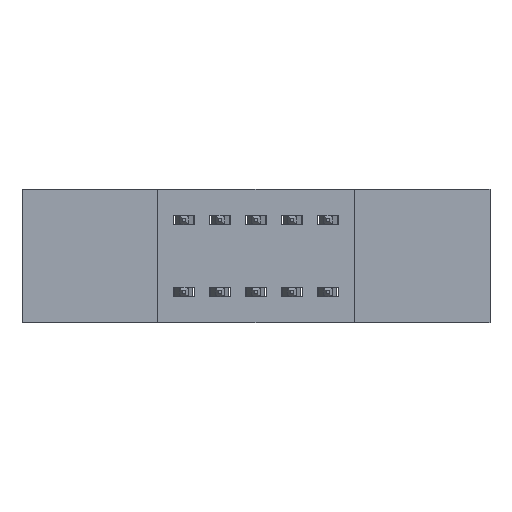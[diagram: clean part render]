
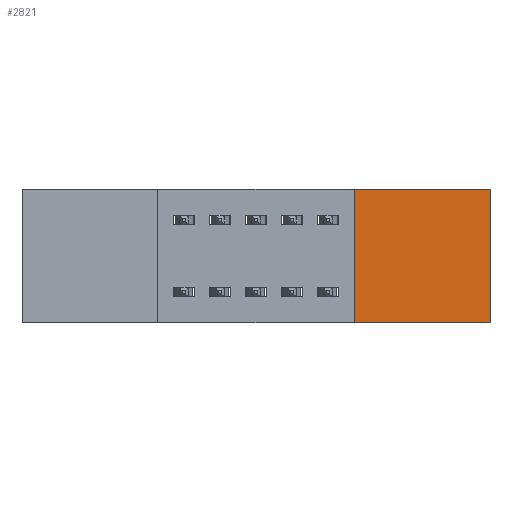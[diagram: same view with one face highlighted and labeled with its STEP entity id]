
A CAD part, front view. The second image highlights one B-rep face of the part: STEP entity #2821.
In plain terms, the highlighted planar face has unit normal (0, -1, 0).
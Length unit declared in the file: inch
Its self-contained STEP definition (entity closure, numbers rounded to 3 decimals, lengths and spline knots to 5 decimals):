
#245 = ORIENTED_EDGE ( 'NONE', *, *, #5132, .F. ) ;
#257 = VECTOR ( 'NONE', #2340, 39.37008 ) ;
#269 = FACE_OUTER_BOUND ( 'NONE', #7204, .T. ) ;
#697 = ORIENTED_EDGE ( 'NONE', *, *, #5958, .F. ) ;
#896 = EDGE_CURVE ( 'NONE', #3418, #1655, #3836, .T. ) ;
#955 = PLANE ( 'NONE',  #3244 ) ;
#995 = CARTESIAN_POINT ( 'NONE',  ( 0., 0., -0.37 ) ) ;
#1147 = VERTEX_POINT ( 'NONE', #1577 ) ;
#1577 = CARTESIAN_POINT ( 'NONE',  ( 0.923, 0., 0. ) ) ;
#1655 = VERTEX_POINT ( 'NONE', #2865 ) ;
#1747 = LINE ( 'NONE', #2254, #7863 ) ;
#2162 = DIRECTION ( 'NONE',  ( 0., -1., 0. ) ) ;
#2254 = CARTESIAN_POINT ( 'NONE',  ( 0., 0., 0. ) ) ;
#2340 = DIRECTION ( 'NONE',  ( 0., 0., -1. ) ) ;
#2496 = CARTESIAN_POINT ( 'NONE',  ( 0., 0., -0.37 ) ) ;
#2521 = ORIENTED_EDGE ( 'NONE', *, *, #4552, .F. ) ;
#2821 = ADVANCED_FACE ( 'NONE', ( #269 ), #955, .T. ) ;
#2865 = CARTESIAN_POINT ( 'NONE',  ( 1.3, 0., -0.37 ) ) ;
#3244 = AXIS2_PLACEMENT_3D ( 'NONE', #2496, #2162, #5313 ) ;
#3418 = VERTEX_POINT ( 'NONE', #5886 ) ;
#3768 = CARTESIAN_POINT ( 'NONE',  ( 0.923, 0., -0.37 ) ) ;
#3836 = LINE ( 'NONE', #4072, #257 ) ;
#4072 = CARTESIAN_POINT ( 'NONE',  ( 1.3, 0., 0. ) ) ;
#4094 = VECTOR ( 'NONE', #7202, 39.37008 ) ;
#4458 = DIRECTION ( 'NONE',  ( 0., 0., 1. ) ) ;
#4552 = EDGE_CURVE ( 'NONE', #1655, #5165, #7311, .T. ) ;
#4996 = VECTOR ( 'NONE', #4458, 39.37008 ) ;
#5132 = EDGE_CURVE ( 'NONE', #1147, #3418, #1747, .T. ) ;
#5165 = VERTEX_POINT ( 'NONE', #3768 ) ;
#5277 = ORIENTED_EDGE ( 'NONE', *, *, #896, .F. ) ;
#5313 = DIRECTION ( 'NONE',  ( 0., 0., -1. ) ) ;
#5513 = DIRECTION ( 'NONE',  ( 1., 0., 0. ) ) ;
#5886 = CARTESIAN_POINT ( 'NONE',  ( 1.3, 0., 0. ) ) ;
#5958 = EDGE_CURVE ( 'NONE', #5165, #1147, #6516, .T. ) ;
#6516 = LINE ( 'NONE', #7181, #4996 ) ;
#7181 = CARTESIAN_POINT ( 'NONE',  ( 0.923, 0., -0.37 ) ) ;
#7202 = DIRECTION ( 'NONE',  ( -1., 0., 0. ) ) ;
#7204 = EDGE_LOOP ( 'NONE', ( #697, #2521, #5277, #245 ) ) ;
#7311 = LINE ( 'NONE', #995, #4094 ) ;
#7863 = VECTOR ( 'NONE', #5513, 39.37008 ) ;
